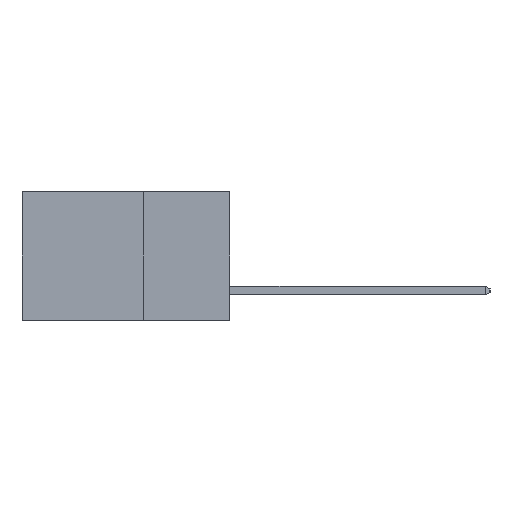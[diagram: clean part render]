
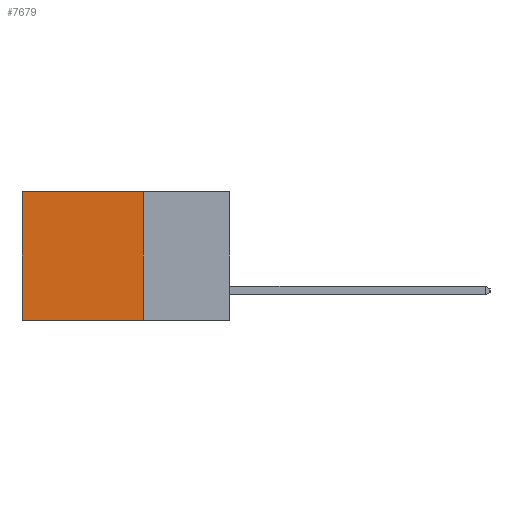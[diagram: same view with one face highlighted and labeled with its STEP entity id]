
A CAD part, left-side view. The second image highlights one B-rep face of the part: STEP entity #7679.
In plain terms, the highlighted planar face has unit normal (-1, 0, 0).
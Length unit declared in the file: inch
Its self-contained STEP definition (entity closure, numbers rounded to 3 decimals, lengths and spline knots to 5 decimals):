
#882 = ORIENTED_EDGE ( 'NONE', *, *, #5894, .F. ) ;
#929 = EDGE_CURVE ( 'NONE', #9903, #1638, #7925, .T. ) ;
#1638 = VERTEX_POINT ( 'NONE', #4157 ) ;
#1875 = EDGE_LOOP ( 'NONE', ( #5691, #882, #10055, #3612 ) ) ;
#1917 = VECTOR ( 'NONE', #6550, 39.37008 ) ;
#2653 = DIRECTION ( 'NONE',  ( 0., 0., -1. ) ) ;
#2863 = VERTEX_POINT ( 'NONE', #3308 ) ;
#3028 = DIRECTION ( 'NONE',  ( 0., 0., -1. ) ) ;
#3271 = DIRECTION ( 'NONE',  ( 0., 1., 0. ) ) ;
#3305 = CARTESIAN_POINT ( 'NONE',  ( 0.298, 0.25, -0.37 ) ) ;
#3308 = CARTESIAN_POINT ( 'NONE',  ( 0.298, 0.25, 0. ) ) ;
#3504 = LINE ( 'NONE', #3305, #3773 ) ;
#3612 = ORIENTED_EDGE ( 'NONE', *, *, #10482, .T. ) ;
#3773 = VECTOR ( 'NONE', #3271, 39.37008 ) ;
#4157 = CARTESIAN_POINT ( 'NONE',  ( 0.298, 0.6, -0.37 ) ) ;
#5644 = CARTESIAN_POINT ( 'NONE',  ( 0.298, 0.25, 0. ) ) ;
#5691 = ORIENTED_EDGE ( 'NONE', *, *, #929, .T. ) ;
#5894 = EDGE_CURVE ( 'NONE', #6374, #1638, #3504, .T. ) ;
#5939 = VECTOR ( 'NONE', #2653, 39.37008 ) ;
#6000 = DIRECTION ( 'NONE',  ( 0., 1., 0. ) ) ;
#6197 = LINE ( 'NONE', #6855, #8176 ) ;
#6363 = AXIS2_PLACEMENT_3D ( 'NONE', #5644, #8203, #3028 ) ;
#6374 = VERTEX_POINT ( 'NONE', #7283 ) ;
#6550 = DIRECTION ( 'NONE',  ( 0., 0., -1. ) ) ;
#6605 = LINE ( 'NONE', #10783, #1917 ) ;
#6825 = CARTESIAN_POINT ( 'NONE',  ( 0.298, 0.6, 0. ) ) ;
#6855 = CARTESIAN_POINT ( 'NONE',  ( 0.298, 0.25, 0. ) ) ;
#7283 = CARTESIAN_POINT ( 'NONE',  ( 0.298, 0.25, -0.37 ) ) ;
#7367 = PLANE ( 'NONE',  #6363 ) ;
#7679 = ADVANCED_FACE ( 'NONE', ( #10018 ), #7367, .F. ) ;
#7885 = CARTESIAN_POINT ( 'NONE',  ( 0.298, 0.6, 0. ) ) ;
#7925 = LINE ( 'NONE', #7885, #5939 ) ;
#8176 = VECTOR ( 'NONE', #6000, 39.37008 ) ;
#8203 = DIRECTION ( 'NONE',  ( 1., 0., 0. ) ) ;
#9903 = VERTEX_POINT ( 'NONE', #6825 ) ;
#10018 = FACE_OUTER_BOUND ( 'NONE', #1875, .T. ) ;
#10055 = ORIENTED_EDGE ( 'NONE', *, *, #10209, .F. ) ;
#10209 = EDGE_CURVE ( 'NONE', #2863, #6374, #6605, .T. ) ;
#10482 = EDGE_CURVE ( 'NONE', #2863, #9903, #6197, .T. ) ;
#10783 = CARTESIAN_POINT ( 'NONE',  ( 0.298, 0.25, 0. ) ) ;
